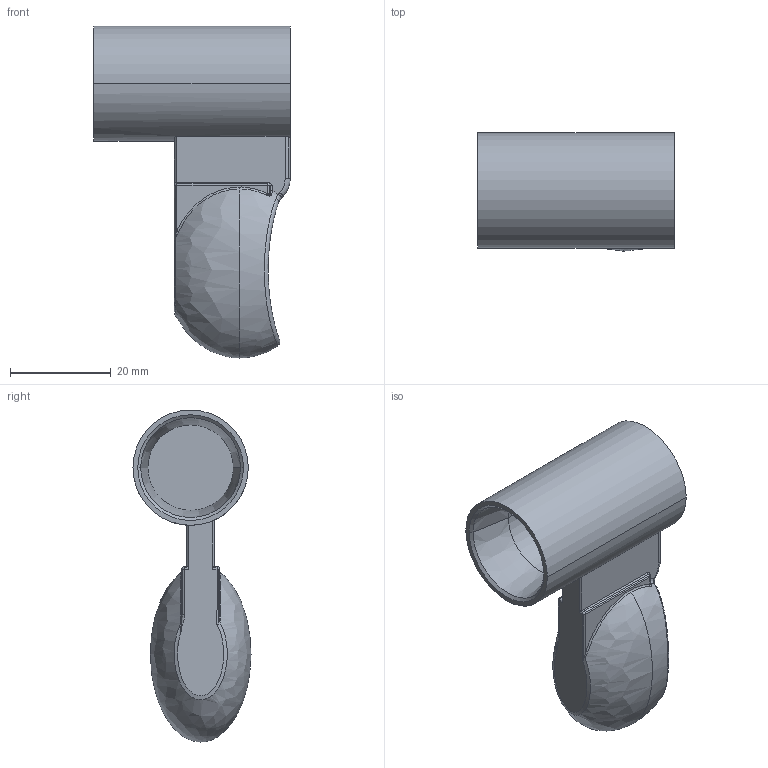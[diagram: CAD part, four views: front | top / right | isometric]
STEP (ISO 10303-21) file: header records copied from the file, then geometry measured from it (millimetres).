
FILE_DESCRIPTION(('STEP AP214'),'1');
FILE_NAME('Charging handle mod 2.stp','2020-08-06T23:43:16',(' '),(' '),'Spatial InterOp 3D',' ',' ');
FILE_SCHEMA(('AUTOMOTIVE_DESIGN { 1 0 10303 214 1 1 1 1 }'));
Length unit declared in the file: metre
Products named in the file (1): Solid1
Bounding box: 39 x 23.45 x 65.95 mm (x, y, z)
Volume: 19931.4 mm3; surface area: 7533.3 mm2
Topology: 1 solids, 1 shells, 77 faces, 197 edges, 120 vertices
Faces by surface type: bspline 29, cylinder 24, plane 16, cone 4, sphere 4
Entity records: 7134 total; most frequent: CARTESIAN_POINT 5406, ORIENTED_EDGE 386, DIRECTION 316, EDGE_CURVE 193, AXIS2_PLACEMENT_3D 132, VERTEX_POINT 120, EDGE_LOOP 79, ADVANCED_FACE 77
